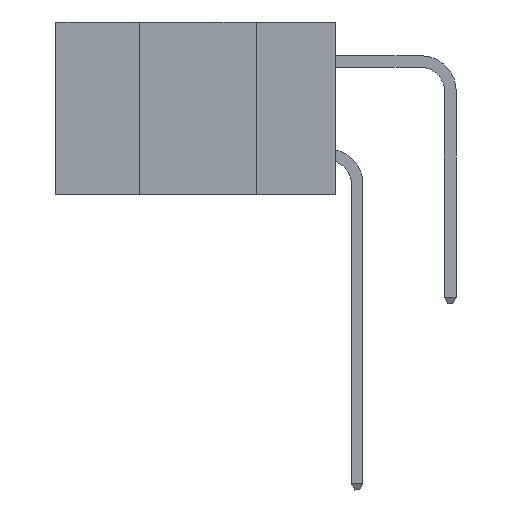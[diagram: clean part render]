
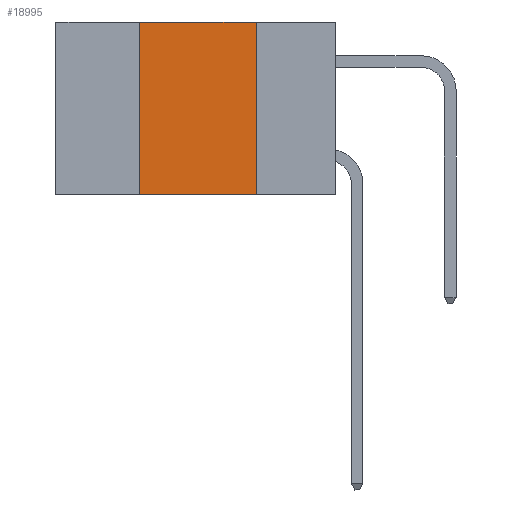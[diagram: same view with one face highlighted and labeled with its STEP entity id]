
A CAD part, left-side view. The second image highlights one B-rep face of the part: STEP entity #18995.
In plain terms, the highlighted planar face has unit normal (-1, 0, 0).
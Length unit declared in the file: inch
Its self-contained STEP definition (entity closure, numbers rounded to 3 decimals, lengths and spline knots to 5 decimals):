
#67 = DIRECTION ( 'NONE',  ( 0., -1., 0. ) ) ;
#351 = VERTEX_POINT ( 'NONE', #12704 ) ;
#1308 = CARTESIAN_POINT ( 'NONE',  ( 0., 0.6, 0. ) ) ;
#1340 = LINE ( 'NONE', #13365, #2481 ) ;
#2143 = CARTESIAN_POINT ( 'NONE',  ( 0., 0.42, 0. ) ) ;
#2264 = AXIS2_PLACEMENT_3D ( 'NONE', #5256, #3441, #16428 ) ;
#2481 = VECTOR ( 'NONE', #7670, 39.37008 ) ;
#3441 = DIRECTION ( 'NONE',  ( 1., 0., 0. ) ) ;
#5107 = VECTOR ( 'NONE', #6908, 39.37008 ) ;
#5238 = DIRECTION ( 'NONE',  ( 0., 0., 1. ) ) ;
#5256 = CARTESIAN_POINT ( 'NONE',  ( 0., 0.6, 0. ) ) ;
#5400 = ORIENTED_EDGE ( 'NONE', *, *, #10566, .F. ) ;
#6300 = LINE ( 'NONE', #1308, #5107 ) ;
#6908 = DIRECTION ( 'NONE',  ( 0., -1., 0. ) ) ;
#7268 = VECTOR ( 'NONE', #5238, 39.37008 ) ;
#7670 = DIRECTION ( 'NONE',  ( 0., 0., -1. ) ) ;
#9456 = LINE ( 'NONE', #11333, #14334 ) ;
#10566 = EDGE_CURVE ( 'NONE', #20379, #17037, #6300, .T. ) ;
#11333 = CARTESIAN_POINT ( 'NONE',  ( 0., 0.6, -0.37 ) ) ;
#12553 = CARTESIAN_POINT ( 'NONE',  ( 0., 0.17, 0. ) ) ;
#12704 = CARTESIAN_POINT ( 'NONE',  ( 0., 0.42, -0.37 ) ) ;
#13365 = CARTESIAN_POINT ( 'NONE',  ( 0., 0.17, 0. ) ) ;
#13949 = EDGE_LOOP ( 'NONE', ( #14205, #5400, #16970, #22218 ) ) ;
#14205 = ORIENTED_EDGE ( 'NONE', *, *, #21881, .F. ) ;
#14334 = VECTOR ( 'NONE', #67, 39.37008 ) ;
#14664 = PLANE ( 'NONE',  #2264 ) ;
#15927 = EDGE_CURVE ( 'NONE', #351, #16569, #9456, .T. ) ;
#16428 = DIRECTION ( 'NONE',  ( 0., 0., -1. ) ) ;
#16482 = LINE ( 'NONE', #21604, #7268 ) ;
#16569 = VERTEX_POINT ( 'NONE', #20085 ) ;
#16970 = ORIENTED_EDGE ( 'NONE', *, *, #17136, .F. ) ;
#17037 = VERTEX_POINT ( 'NONE', #12553 ) ;
#17136 = EDGE_CURVE ( 'NONE', #351, #20379, #16482, .T. ) ;
#18995 = ADVANCED_FACE ( 'NONE', ( #19466 ), #14664, .F. ) ;
#19466 = FACE_OUTER_BOUND ( 'NONE', #13949, .T. ) ;
#20085 = CARTESIAN_POINT ( 'NONE',  ( 0., 0.17, -0.37 ) ) ;
#20379 = VERTEX_POINT ( 'NONE', #2143 ) ;
#21604 = CARTESIAN_POINT ( 'NONE',  ( 0., 0.42, 0. ) ) ;
#21881 = EDGE_CURVE ( 'NONE', #17037, #16569, #1340, .T. ) ;
#22218 = ORIENTED_EDGE ( 'NONE', *, *, #15927, .T. ) ;
